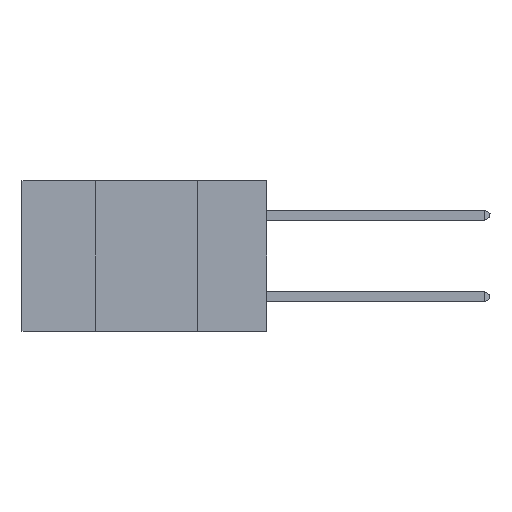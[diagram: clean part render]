
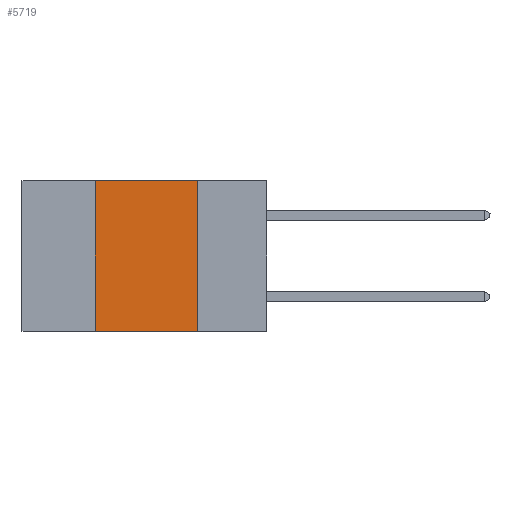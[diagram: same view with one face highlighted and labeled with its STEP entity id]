
A CAD part, left-side view. The second image highlights one B-rep face of the part: STEP entity #5719.
In plain terms, the highlighted planar face has unit normal (-1, 0, 0).
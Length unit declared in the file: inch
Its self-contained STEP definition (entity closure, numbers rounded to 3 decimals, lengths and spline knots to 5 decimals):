
#26 = ORIENTED_EDGE ( 'NONE', *, *, #9833, .T. ) ;
#123 = CARTESIAN_POINT ( 'NONE',  ( 0., 0.42, 0. ) ) ;
#190 = CARTESIAN_POINT ( 'NONE',  ( 0., 0.6, 0. ) ) ;
#295 = ORIENTED_EDGE ( 'NONE', *, *, #1341, .F. ) ;
#1153 = DIRECTION ( 'NONE',  ( 0., -1., 0. ) ) ;
#1341 = EDGE_CURVE ( 'NONE', #3728, #10362, #10186, .T. ) ;
#1676 = CARTESIAN_POINT ( 'NONE',  ( 0., 0.17, 0. ) ) ;
#1695 = EDGE_LOOP ( 'NONE', ( #8572, #295, #10921, #26 ) ) ;
#1863 = VECTOR ( 'NONE', #4244, 39.37008 ) ;
#1945 = VECTOR ( 'NONE', #2103, 39.37008 ) ;
#2103 = DIRECTION ( 'NONE',  ( 0., -1., 0. ) ) ;
#2281 = VECTOR ( 'NONE', #2531, 39.37008 ) ;
#2317 = PLANE ( 'NONE',  #6634 ) ;
#2531 = DIRECTION ( 'NONE',  ( 0., 0., -1. ) ) ;
#3450 = CARTESIAN_POINT ( 'NONE',  ( 0., 0.17, 0. ) ) ;
#3698 = CARTESIAN_POINT ( 'NONE',  ( 0., 0.6, -0.37 ) ) ;
#3728 = VERTEX_POINT ( 'NONE', #123 ) ;
#4093 = DIRECTION ( 'NONE',  ( 1., 0., 0. ) ) ;
#4244 = DIRECTION ( 'NONE',  ( 0., 0., 1. ) ) ;
#4263 = VECTOR ( 'NONE', #1153, 39.37008 ) ;
#4317 = CARTESIAN_POINT ( 'NONE',  ( 0., 0.42, 0. ) ) ;
#4391 = LINE ( 'NONE', #1676, #2281 ) ;
#4439 = CARTESIAN_POINT ( 'NONE',  ( 0., 0.17, -0.37 ) ) ;
#4522 = CARTESIAN_POINT ( 'NONE',  ( 0., 0.42, -0.37 ) ) ;
#5326 = LINE ( 'NONE', #4317, #1863 ) ;
#5365 = VERTEX_POINT ( 'NONE', #4522 ) ;
#5719 = ADVANCED_FACE ( 'NONE', ( #10802 ), #2317, .F. ) ;
#5795 = DIRECTION ( 'NONE',  ( 0., 0., -1. ) ) ;
#5908 = LINE ( 'NONE', #3698, #4263 ) ;
#6634 = AXIS2_PLACEMENT_3D ( 'NONE', #10841, #4093, #5795 ) ;
#8137 = VERTEX_POINT ( 'NONE', #4439 ) ;
#8572 = ORIENTED_EDGE ( 'NONE', *, *, #9696, .F. ) ;
#8574 = EDGE_CURVE ( 'NONE', #5365, #3728, #5326, .T. ) ;
#9696 = EDGE_CURVE ( 'NONE', #10362, #8137, #4391, .T. ) ;
#9833 = EDGE_CURVE ( 'NONE', #5365, #8137, #5908, .T. ) ;
#10186 = LINE ( 'NONE', #190, #1945 ) ;
#10362 = VERTEX_POINT ( 'NONE', #3450 ) ;
#10802 = FACE_OUTER_BOUND ( 'NONE', #1695, .T. ) ;
#10841 = CARTESIAN_POINT ( 'NONE',  ( 0., 0.6, 0. ) ) ;
#10921 = ORIENTED_EDGE ( 'NONE', *, *, #8574, .F. ) ;
